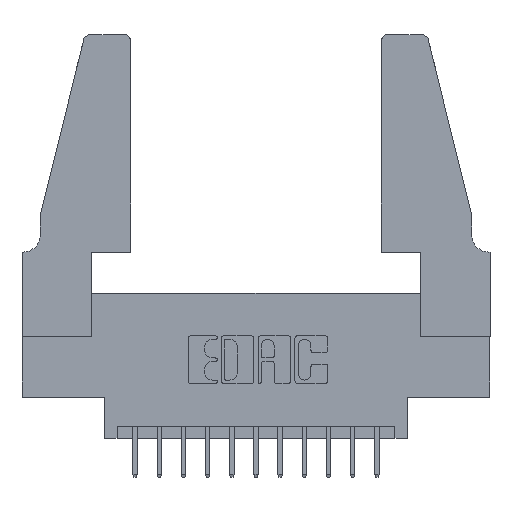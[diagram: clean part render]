
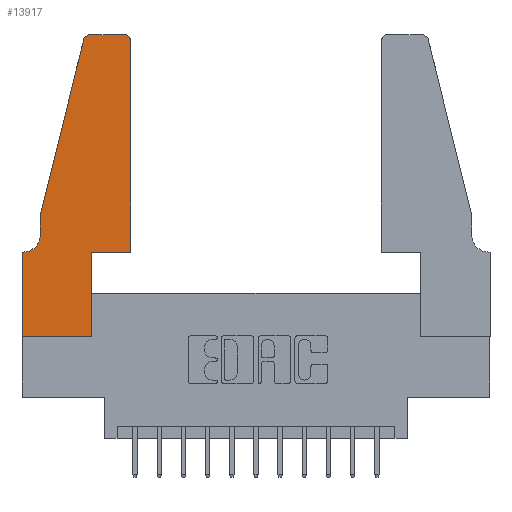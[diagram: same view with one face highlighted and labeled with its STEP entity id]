
A CAD part, top view. The second image highlights one B-rep face of the part: STEP entity #13917.
In plain terms, the highlighted planar face has unit normal (0, 0, 1).
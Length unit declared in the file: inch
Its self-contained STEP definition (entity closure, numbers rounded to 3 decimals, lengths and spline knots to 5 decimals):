
#346 = CARTESIAN_POINT ( 'NONE',  ( 0.4505, 0.35, 0.37 ) ) ;
#468 = VECTOR ( 'NONE', #14143, 39.37008 ) ;
#592 = CARTESIAN_POINT ( 'NONE',  ( 0.4505, 1.22, 0.37 ) ) ;
#984 = VECTOR ( 'NONE', #9711, 39.37008 ) ;
#1086 = DIRECTION ( 'NONE',  ( 1., 0., 0. ) ) ;
#1129 = VECTOR ( 'NONE', #2002, 39.37008 ) ;
#1206 = CARTESIAN_POINT ( 'NONE',  ( 0., 0.35, 0.37 ) ) ;
#1304 = LINE ( 'NONE', #6755, #13711 ) ;
#1322 = ORIENTED_EDGE ( 'NONE', *, *, #2354, .T. ) ;
#1379 = LINE ( 'NONE', #14289, #984 ) ;
#1585 = DIRECTION ( 'NONE',  ( 0., 1., 0. ) ) ;
#1883 = VERTEX_POINT ( 'NONE', #7915 ) ;
#2002 = DIRECTION ( 'NONE',  ( -0.239, -0.971, 0. ) ) ;
#2354 = EDGE_CURVE ( 'NONE', #14131, #4004, #13563, .T. ) ;
#2568 = ORIENTED_EDGE ( 'NONE', *, *, #4877, .T. ) ;
#2602 = CARTESIAN_POINT ( 'NONE',  ( 0.2865, 0., 0.37 ) ) ;
#2707 = LINE ( 'NONE', #10329, #11228 ) ;
#2854 = LINE ( 'NONE', #9252, #5941 ) ;
#2930 = EDGE_CURVE ( 'NONE', #4004, #4526, #2854, .T. ) ;
#2997 = AXIS2_PLACEMENT_3D ( 'NONE', #5248, #6391, #14478 ) ;
#3478 = VERTEX_POINT ( 'NONE', #11692 ) ;
#3608 = VERTEX_POINT ( 'NONE', #4312 ) ;
#3732 = EDGE_CURVE ( 'NONE', #7265, #13628, #6980, .T. ) ;
#3758 = VECTOR ( 'NONE', #1086, 39.37008 ) ;
#3965 = EDGE_CURVE ( 'NONE', #13628, #13085, #4115, .T. ) ;
#4004 = VERTEX_POINT ( 'NONE', #6636 ) ;
#4094 = PLANE ( 'NONE',  #2997 ) ;
#4115 = LINE ( 'NONE', #8358, #3758 ) ;
#4303 = CARTESIAN_POINT ( 'NONE',  ( 0.284, 1.22, 0.37 ) ) ;
#4312 = CARTESIAN_POINT ( 'NONE',  ( 0.4205, 1.25, 0.37 ) ) ;
#4437 = DIRECTION ( 'NONE',  ( 0., 0., -1. ) ) ;
#4526 = VERTEX_POINT ( 'NONE', #7708 ) ;
#4690 = ORIENTED_EDGE ( 'NONE', *, *, #2930, .T. ) ;
#4847 = FACE_OUTER_BOUND ( 'NONE', #14413, .T. ) ;
#4877 = EDGE_CURVE ( 'NONE', #13085, #14568, #12585, .T. ) ;
#5231 = CARTESIAN_POINT ( 'NONE',  ( 0.4505, 0.35, 0.37 ) ) ;
#5248 = CARTESIAN_POINT ( 'NONE',  ( 0., 0.35, 0.37 ) ) ;
#5264 = ORIENTED_EDGE ( 'NONE', *, *, #14076, .T. ) ;
#5453 = DIRECTION ( 'NONE',  ( 1., 0., 0. ) ) ;
#5941 = VECTOR ( 'NONE', #8201, 39.37008 ) ;
#6235 = CARTESIAN_POINT ( 'NONE',  ( 0.4205, 1.22, 0.37 ) ) ;
#6391 = DIRECTION ( 'NONE',  ( 0., 0., 1. ) ) ;
#6573 = ORIENTED_EDGE ( 'NONE', *, *, #3965, .T. ) ;
#6636 = CARTESIAN_POINT ( 'NONE',  ( 0.0755, 0.5, 0.37 ) ) ;
#6755 = CARTESIAN_POINT ( 'NONE',  ( 0.2605, 1.25, 0.37 ) ) ;
#6787 = ORIENTED_EDGE ( 'NONE', *, *, #11960, .T. ) ;
#6980 = LINE ( 'NONE', #10460, #10084 ) ;
#7053 = CIRCLE ( 'NONE', #13982, 0.03 ) ;
#7062 = ORIENTED_EDGE ( 'NONE', *, *, #14861, .T. ) ;
#7265 = VERTEX_POINT ( 'NONE', #1206 ) ;
#7300 = LINE ( 'NONE', #346, #13125 ) ;
#7379 = DIRECTION ( 'NONE',  ( 1., 0., 0. ) ) ;
#7421 = ORIENTED_EDGE ( 'NONE', *, *, #3732, .T. ) ;
#7523 = CARTESIAN_POINT ( 'NONE',  ( 0.2865, 0.35, 0.37 ) ) ;
#7646 = EDGE_CURVE ( 'NONE', #1883, #14131, #7053, .T. ) ;
#7708 = CARTESIAN_POINT ( 'NONE',  ( 0.0755, 0.42, 0.37 ) ) ;
#7765 = CIRCLE ( 'NONE', #9686, 0.03 ) ;
#7915 = CARTESIAN_POINT ( 'NONE',  ( 0.284, 1.25, 0.37 ) ) ;
#8201 = DIRECTION ( 'NONE',  ( 0., -1., 0. ) ) ;
#8358 = CARTESIAN_POINT ( 'NONE',  ( 0., 0., 0.37 ) ) ;
#8813 = EDGE_CURVE ( 'NONE', #12068, #13967, #7300, .T. ) ;
#9252 = CARTESIAN_POINT ( 'NONE',  ( 0.0755, 0.5, 0.37 ) ) ;
#9686 = AXIS2_PLACEMENT_3D ( 'NONE', #6235, #14322, #7379 ) ;
#9711 = DIRECTION ( 'NONE',  ( 1., 0., 0. ) ) ;
#10084 = VECTOR ( 'NONE', #13088, 39.37008 ) ;
#10303 = ORIENTED_EDGE ( 'NONE', *, *, #7646, .T. ) ;
#10329 = CARTESIAN_POINT ( 'NONE',  ( 0.0755, 0.35, 0.37 ) ) ;
#10460 = CARTESIAN_POINT ( 'NONE',  ( 0., 0., 0.37 ) ) ;
#10567 = ORIENTED_EDGE ( 'NONE', *, *, #11314, .T. ) ;
#10763 = AXIS2_PLACEMENT_3D ( 'NONE', #11360, #4437, #12535 ) ;
#11228 = VECTOR ( 'NONE', #13811, 39.37008 ) ;
#11314 = EDGE_CURVE ( 'NONE', #14568, #12068, #1379, .T. ) ;
#11360 = CARTESIAN_POINT ( 'NONE',  ( 0.0055, 0.42, 0.37 ) ) ;
#11456 = CARTESIAN_POINT ( 'NONE',  ( 0.0755, 0.5, 0.37 ) ) ;
#11531 = CIRCLE ( 'NONE', #10763, 0.07 ) ;
#11692 = CARTESIAN_POINT ( 'NONE',  ( 0.0055, 0.35, 0.37 ) ) ;
#11960 = EDGE_CURVE ( 'NONE', #13967, #3608, #7765, .T. ) ;
#11961 = ORIENTED_EDGE ( 'NONE', *, *, #8813, .T. ) ;
#12068 = VERTEX_POINT ( 'NONE', #5231 ) ;
#12396 = DIRECTION ( 'NONE',  ( 0., 0., 1. ) ) ;
#12443 = ORIENTED_EDGE ( 'NONE', *, *, #13458, .T. ) ;
#12535 = DIRECTION ( 'NONE',  ( -1., 0., 0. ) ) ;
#12585 = LINE ( 'NONE', #13000, #468 ) ;
#12844 = CARTESIAN_POINT ( 'NONE',  ( 0., 0., 0.37 ) ) ;
#13000 = CARTESIAN_POINT ( 'NONE',  ( 0.2865, 0.35, 0.37 ) ) ;
#13085 = VERTEX_POINT ( 'NONE', #2602 ) ;
#13088 = DIRECTION ( 'NONE',  ( 0., -1., 0. ) ) ;
#13125 = VECTOR ( 'NONE', #1585, 39.37008 ) ;
#13458 = EDGE_CURVE ( 'NONE', #3608, #1883, #1304, .T. ) ;
#13563 = LINE ( 'NONE', #11456, #1129 ) ;
#13628 = VERTEX_POINT ( 'NONE', #12844 ) ;
#13711 = VECTOR ( 'NONE', #14842, 39.37008 ) ;
#13727 = CARTESIAN_POINT ( 'NONE',  ( 0.25487, 1.22718, 0.37 ) ) ;
#13811 = DIRECTION ( 'NONE',  ( -1., 0., 0. ) ) ;
#13917 = ADVANCED_FACE ( 'NONE', ( #4847 ), #4094, .T. ) ;
#13967 = VERTEX_POINT ( 'NONE', #592 ) ;
#13982 = AXIS2_PLACEMENT_3D ( 'NONE', #4303, #12396, #5453 ) ;
#14076 = EDGE_CURVE ( 'NONE', #4526, #3478, #11531, .T. ) ;
#14131 = VERTEX_POINT ( 'NONE', #13727 ) ;
#14143 = DIRECTION ( 'NONE',  ( 0., 1., 0. ) ) ;
#14289 = CARTESIAN_POINT ( 'NONE',  ( 0.4505, 0.35, 0.37 ) ) ;
#14322 = DIRECTION ( 'NONE',  ( 0., 0., 1. ) ) ;
#14413 = EDGE_LOOP ( 'NONE', ( #12443, #10303, #1322, #4690, #5264, #7062, #7421, #6573, #2568, #10567, #11961, #6787 ) ) ;
#14478 = DIRECTION ( 'NONE',  ( 1., 0., 0. ) ) ;
#14568 = VERTEX_POINT ( 'NONE', #7523 ) ;
#14842 = DIRECTION ( 'NONE',  ( -1., 0., 0. ) ) ;
#14861 = EDGE_CURVE ( 'NONE', #3478, #7265, #2707, .T. ) ;
